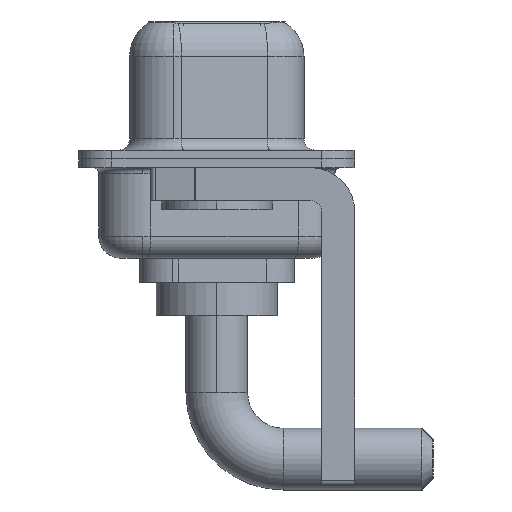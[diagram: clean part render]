
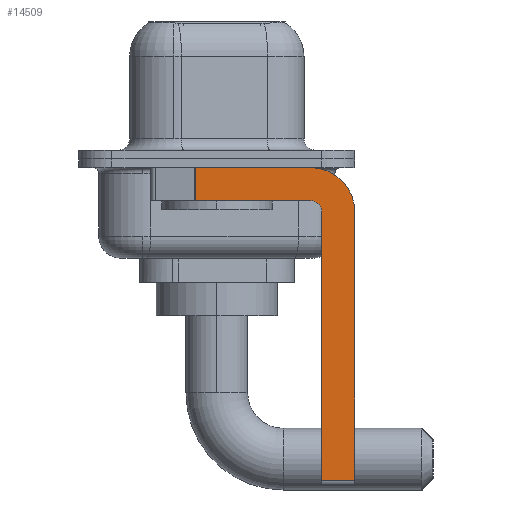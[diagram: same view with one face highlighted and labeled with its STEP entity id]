
A CAD part, left-side view. The second image highlights one B-rep face of the part: STEP entity #14509.
In plain terms, the highlighted planar face has unit normal (-1, 0, 0).
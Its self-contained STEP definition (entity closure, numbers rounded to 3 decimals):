
#143 = CARTESIAN_POINT ( 'NONE',  ( -2.9, -6.25, -14.55 ) ) ;
#167 = VERTEX_POINT ( 'NONE', #10713 ) ;
#493 = DIRECTION ( 'NONE',  ( 1., 0., 0. ) ) ;
#642 = DIRECTION ( 'NONE',  ( 0., 0., -1. ) ) ;
#850 = VERTEX_POINT ( 'NONE', #13557 ) ;
#1236 = AXIS2_PLACEMENT_3D ( 'NONE', #9581, #5345, #11843 ) ;
#1625 = CARTESIAN_POINT ( 'NONE',  ( -2.9, -6.25, -2.4 ) ) ;
#1745 = VERTEX_POINT ( 'NONE', #6872 ) ;
#1970 = EDGE_CURVE ( 'NONE', #167, #12633, #7435, .T. ) ;
#2018 = EDGE_LOOP ( 'NONE', ( #2234, #7378, #3710, #10626, #13244, #7096, #7431, #12007 ) ) ;
#2234 = ORIENTED_EDGE ( 'NONE', *, *, #5284, .F. ) ;
#2312 = CARTESIAN_POINT ( 'NONE',  ( -2.9, -4.25, -1.9 ) ) ;
#2322 = VECTOR ( 'NONE', #10596, 1000. ) ;
#2404 = VERTEX_POINT ( 'NONE', #6767 ) ;
#2458 = LINE ( 'NONE', #2312, #9904 ) ;
#2579 = CARTESIAN_POINT ( 'NONE',  ( -2.9, -4.75, -14.8 ) ) ;
#2773 = DIRECTION ( 'NONE',  ( 0., -1., 0. ) ) ;
#2798 = DIRECTION ( 'NONE',  ( 0., 0., -1. ) ) ;
#3352 = VECTOR ( 'NONE', #2773, 1000. ) ;
#3710 = ORIENTED_EDGE ( 'NONE', *, *, #4142, .F. ) ;
#4142 = EDGE_CURVE ( 'NONE', #850, #12633, #2458, .T. ) ;
#4818 = VECTOR ( 'NONE', #12481, 1000. ) ;
#4926 = LINE ( 'NONE', #1625, #2322 ) ;
#5027 = EDGE_CURVE ( 'NONE', #1745, #850, #5435, .T. ) ;
#5284 = EDGE_CURVE ( 'NONE', #167, #2404, #7159, .T. ) ;
#5345 = DIRECTION ( 'NONE',  ( -1., 0., 0. ) ) ;
#5435 = CIRCLE ( 'NONE', #1236, 0.5 ) ;
#6311 = VECTOR ( 'NONE', #7048, 1000. ) ;
#6640 = CARTESIAN_POINT ( 'NONE',  ( -2.9, -6.25, -2.4 ) ) ;
#6767 = CARTESIAN_POINT ( 'NONE',  ( -2.9, -4.25, -0.4 ) ) ;
#6777 = DIRECTION ( 'NONE',  ( 0., 1., 0. ) ) ;
#6855 = VECTOR ( 'NONE', #12012, 1000. ) ;
#6872 = CARTESIAN_POINT ( 'NONE',  ( -2.9, -4.75, -2.4 ) ) ;
#7048 = DIRECTION ( 'NONE',  ( 0., 0., 1. ) ) ;
#7096 = ORIENTED_EDGE ( 'NONE', *, *, #7692, .T. ) ;
#7159 = LINE ( 'NONE', #8417, #3352 ) ;
#7378 = ORIENTED_EDGE ( 'NONE', *, *, #1970, .T. ) ;
#7431 = ORIENTED_EDGE ( 'NONE', *, *, #12864, .F. ) ;
#7435 = LINE ( 'NONE', #8616, #6855 ) ;
#7692 = EDGE_CURVE ( 'NONE', #11402, #13779, #12716, .T. ) ;
#8375 = CARTESIAN_POINT ( 'NONE',  ( -2.9, -4.25, -2.4 ) ) ;
#8417 = CARTESIAN_POINT ( 'NONE',  ( -2.9, 3., -0.4 ) ) ;
#8616 = CARTESIAN_POINT ( 'NONE',  ( -2.9, 0.978, -1.9 ) ) ;
#8819 = CARTESIAN_POINT ( 'NONE',  ( -2.9, -4.75, -14.55 ) ) ;
#9401 = CARTESIAN_POINT ( 'NONE',  ( -2.9, -4.25, -14.55 ) ) ;
#9581 = CARTESIAN_POINT ( 'NONE',  ( -2.9, -4.25, -2.4 ) ) ;
#9680 = CARTESIAN_POINT ( 'NONE',  ( -2.9, -4.25, -2.4 ) ) ;
#9849 = AXIS2_PLACEMENT_3D ( 'NONE', #9680, #493, #642 ) ;
#9904 = VECTOR ( 'NONE', #6777, 1000. ) ;
#10013 = CARTESIAN_POINT ( 'NONE',  ( -2.9, 0.978, -1.9 ) ) ;
#10016 = AXIS2_PLACEMENT_3D ( 'NONE', #8375, #12879, #2798 ) ;
#10409 = EDGE_CURVE ( 'NONE', #2404, #12252, #10955, .T. ) ;
#10570 = PLANE ( 'NONE',  #9849 ) ;
#10596 = DIRECTION ( 'NONE',  ( 0., 0., -1. ) ) ;
#10626 = ORIENTED_EDGE ( 'NONE', *, *, #5027, .F. ) ;
#10713 = CARTESIAN_POINT ( 'NONE',  ( -2.9, 0.978, -0.4 ) ) ;
#10955 = CIRCLE ( 'NONE', #10016, 2. ) ;
#11402 = VERTEX_POINT ( 'NONE', #8819 ) ;
#11843 = DIRECTION ( 'NONE',  ( 0., 0., 1. ) ) ;
#12007 = ORIENTED_EDGE ( 'NONE', *, *, #10409, .F. ) ;
#12012 = DIRECTION ( 'NONE',  ( 0., 0., -1. ) ) ;
#12252 = VERTEX_POINT ( 'NONE', #6640 ) ;
#12481 = DIRECTION ( 'NONE',  ( 0., -1., 0. ) ) ;
#12633 = VERTEX_POINT ( 'NONE', #10013 ) ;
#12716 = LINE ( 'NONE', #9401, #4818 ) ;
#12864 = EDGE_CURVE ( 'NONE', #12252, #13779, #4926, .T. ) ;
#12879 = DIRECTION ( 'NONE',  ( 1., 0., 0. ) ) ;
#13244 = ORIENTED_EDGE ( 'NONE', *, *, #13488, .F. ) ;
#13488 = EDGE_CURVE ( 'NONE', #11402, #1745, #13920, .T. ) ;
#13557 = CARTESIAN_POINT ( 'NONE',  ( -2.9, -4.25, -1.9 ) ) ;
#13779 = VERTEX_POINT ( 'NONE', #143 ) ;
#13920 = LINE ( 'NONE', #2579, #6311 ) ;
#14249 = FACE_OUTER_BOUND ( 'NONE', #2018, .T. ) ;
#14509 = ADVANCED_FACE ( 'NONE', ( #14249 ), #10570, .F. ) ;
